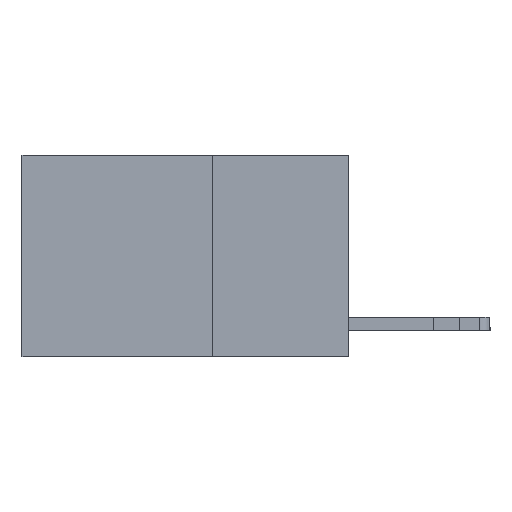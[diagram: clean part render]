
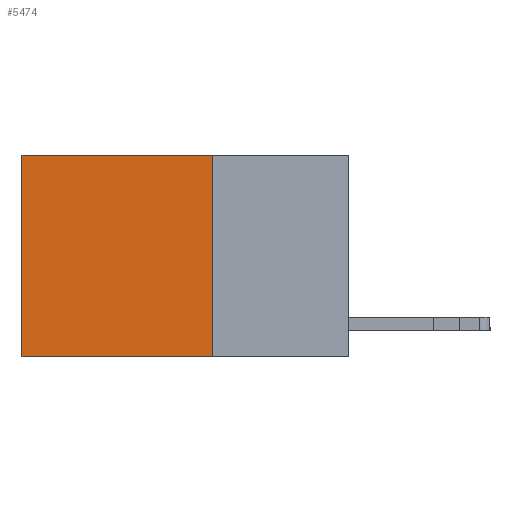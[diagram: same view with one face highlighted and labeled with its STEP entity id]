
A CAD part, left-side view. The second image highlights one B-rep face of the part: STEP entity #5474.
In plain terms, the highlighted planar face has unit normal (-1, 0, 0).
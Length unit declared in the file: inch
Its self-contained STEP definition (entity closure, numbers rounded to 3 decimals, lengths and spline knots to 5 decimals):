
#231 = CARTESIAN_POINT ( 'NONE',  ( 0.2625, 0.25, 0. ) ) ;
#445 = LINE ( 'NONE', #9325, #3745 ) ;
#871 = CARTESIAN_POINT ( 'NONE',  ( 0.2625, 0.6, -0.37 ) ) ;
#1116 = VECTOR ( 'NONE', #8985, 39.37008 ) ;
#1204 = EDGE_LOOP ( 'NONE', ( #5816, #12399, #9305, #6577 ) ) ;
#3745 = VECTOR ( 'NONE', #7411, 39.37008 ) ;
#4083 = LINE ( 'NONE', #231, #1116 ) ;
#4319 = CARTESIAN_POINT ( 'NONE',  ( 0.2625, 0.25, 0. ) ) ;
#4567 = EDGE_CURVE ( 'NONE', #5430, #9004, #445, .T. ) ;
#4879 = CARTESIAN_POINT ( 'NONE',  ( 0.2625, 0.6, 0. ) ) ;
#5024 = CARTESIAN_POINT ( 'NONE',  ( 0.2625, 0.6, 0. ) ) ;
#5092 = DIRECTION ( 'NONE',  ( 1., 0., 0. ) ) ;
#5274 = FACE_OUTER_BOUND ( 'NONE', #1204, .T. ) ;
#5430 = VERTEX_POINT ( 'NONE', #11085 ) ;
#5474 = ADVANCED_FACE ( 'NONE', ( #5274 ), #10967, .F. ) ;
#5816 = ORIENTED_EDGE ( 'NONE', *, *, #10945, .T. ) ;
#6577 = ORIENTED_EDGE ( 'NONE', *, *, #7785, .T. ) ;
#6631 = LINE ( 'NONE', #7780, #11730 ) ;
#7411 = DIRECTION ( 'NONE',  ( 0., 1., 0. ) ) ;
#7780 = CARTESIAN_POINT ( 'NONE',  ( 0.2625, 0.25, 0. ) ) ;
#7785 = EDGE_CURVE ( 'NONE', #10156, #10459, #4083, .T. ) ;
#7807 = LINE ( 'NONE', #4879, #8461 ) ;
#8333 = CARTESIAN_POINT ( 'NONE',  ( 0.2625, 0.25, 0. ) ) ;
#8461 = VECTOR ( 'NONE', #10872, 39.37008 ) ;
#8985 = DIRECTION ( 'NONE',  ( 0., 1., 0. ) ) ;
#9004 = VERTEX_POINT ( 'NONE', #871 ) ;
#9240 = AXIS2_PLACEMENT_3D ( 'NONE', #4319, #5092, #10191 ) ;
#9305 = ORIENTED_EDGE ( 'NONE', *, *, #11174, .F. ) ;
#9325 = CARTESIAN_POINT ( 'NONE',  ( 0.2625, 0.25, -0.37 ) ) ;
#10156 = VERTEX_POINT ( 'NONE', #8333 ) ;
#10191 = DIRECTION ( 'NONE',  ( 0., 0., -1. ) ) ;
#10459 = VERTEX_POINT ( 'NONE', #5024 ) ;
#10718 = DIRECTION ( 'NONE',  ( 0., 0., -1. ) ) ;
#10872 = DIRECTION ( 'NONE',  ( 0., 0., -1. ) ) ;
#10945 = EDGE_CURVE ( 'NONE', #10459, #9004, #7807, .T. ) ;
#10967 = PLANE ( 'NONE',  #9240 ) ;
#11085 = CARTESIAN_POINT ( 'NONE',  ( 0.2625, 0.25, -0.37 ) ) ;
#11174 = EDGE_CURVE ( 'NONE', #10156, #5430, #6631, .T. ) ;
#11730 = VECTOR ( 'NONE', #10718, 39.37008 ) ;
#12399 = ORIENTED_EDGE ( 'NONE', *, *, #4567, .F. ) ;
